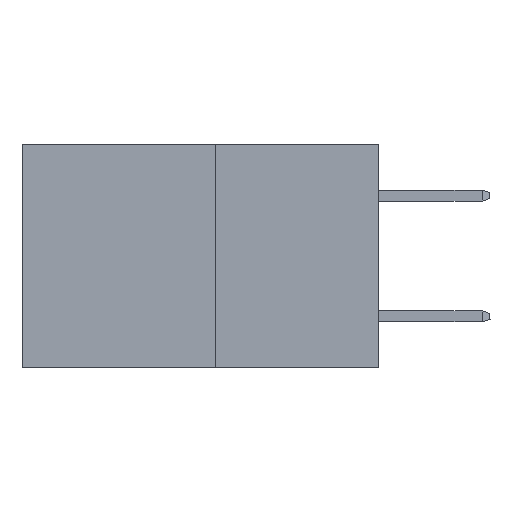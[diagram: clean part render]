
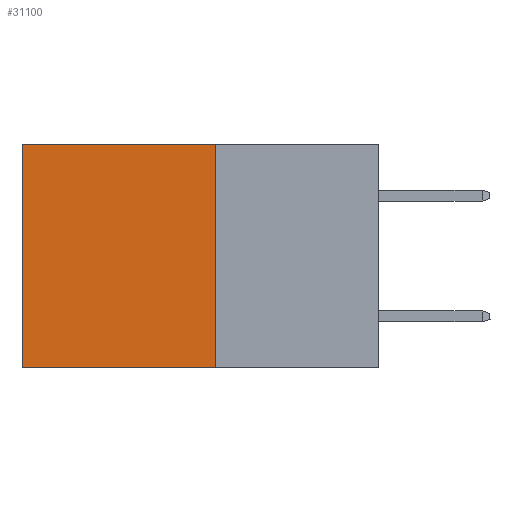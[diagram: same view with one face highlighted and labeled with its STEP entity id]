
A CAD part, left-side view. The second image highlights one B-rep face of the part: STEP entity #31100.
In plain terms, the highlighted planar face has unit normal (-1, 0, 0).
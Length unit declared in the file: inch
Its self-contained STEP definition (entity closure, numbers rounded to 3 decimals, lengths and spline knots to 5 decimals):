
#411 = DIRECTION ( 'NONE',  ( 0., 0., -1. ) ) ;
#451 = CARTESIAN_POINT ( 'NONE',  ( 0.277, 0.59, 0. ) ) ;
#1438 = LINE ( 'NONE', #20582, #20863 ) ;
#2962 = ORIENTED_EDGE ( 'NONE', *, *, #15290, .F. ) ;
#4469 = DIRECTION ( 'NONE',  ( 1., 0., 0. ) ) ;
#5817 = CARTESIAN_POINT ( 'NONE',  ( 0.277, 0.27, -0.37 ) ) ;
#8276 = DIRECTION ( 'NONE',  ( 0., 0., -1. ) ) ;
#8668 = AXIS2_PLACEMENT_3D ( 'NONE', #19058, #4469, #21492 ) ;
#8716 = VERTEX_POINT ( 'NONE', #10966 ) ;
#8997 = VERTEX_POINT ( 'NONE', #9466 ) ;
#9466 = CARTESIAN_POINT ( 'NONE',  ( 0.277, 0.59, -0.37 ) ) ;
#9505 = VECTOR ( 'NONE', #25069, 39.37008 ) ;
#9951 = LINE ( 'NONE', #29394, #22084 ) ;
#10518 = LINE ( 'NONE', #5817, #28206 ) ;
#10966 = CARTESIAN_POINT ( 'NONE',  ( 0.277, 0.27, -0.37 ) ) ;
#11109 = EDGE_LOOP ( 'NONE', ( #13774, #2962, #19157, #23805 ) ) ;
#11236 = VERTEX_POINT ( 'NONE', #451 ) ;
#13263 = DIRECTION ( 'NONE',  ( 0., 1., 0. ) ) ;
#13392 = EDGE_CURVE ( 'NONE', #11236, #8997, #9951, .T. ) ;
#13774 = ORIENTED_EDGE ( 'NONE', *, *, #13392, .T. ) ;
#15290 = EDGE_CURVE ( 'NONE', #8716, #8997, #1438, .T. ) ;
#15963 = LINE ( 'NONE', #20223, #9505 ) ;
#17235 = EDGE_CURVE ( 'NONE', #25312, #8716, #10518, .T. ) ;
#19058 = CARTESIAN_POINT ( 'NONE',  ( 0.277, 0.27, -0.37 ) ) ;
#19157 = ORIENTED_EDGE ( 'NONE', *, *, #17235, .F. ) ;
#20099 = CARTESIAN_POINT ( 'NONE',  ( 0.277, 0.27, 0. ) ) ;
#20223 = CARTESIAN_POINT ( 'NONE',  ( 0.277, 0.27, 0. ) ) ;
#20582 = CARTESIAN_POINT ( 'NONE',  ( 0.277, 0.27, -0.37 ) ) ;
#20863 = VECTOR ( 'NONE', #13263, 39.37008 ) ;
#21492 = DIRECTION ( 'NONE',  ( 0., 0., -1. ) ) ;
#22084 = VECTOR ( 'NONE', #411, 39.37008 ) ;
#23804 = PLANE ( 'NONE',  #8668 ) ;
#23805 = ORIENTED_EDGE ( 'NONE', *, *, #24061, .T. ) ;
#24061 = EDGE_CURVE ( 'NONE', #25312, #11236, #15963, .T. ) ;
#25069 = DIRECTION ( 'NONE',  ( 0., 1., 0. ) ) ;
#25312 = VERTEX_POINT ( 'NONE', #20099 ) ;
#26316 = FACE_OUTER_BOUND ( 'NONE', #11109, .T. ) ;
#28206 = VECTOR ( 'NONE', #8276, 39.37008 ) ;
#29394 = CARTESIAN_POINT ( 'NONE',  ( 0.277, 0.59, -0.37 ) ) ;
#31100 = ADVANCED_FACE ( 'NONE', ( #26316 ), #23804, .F. ) ;
